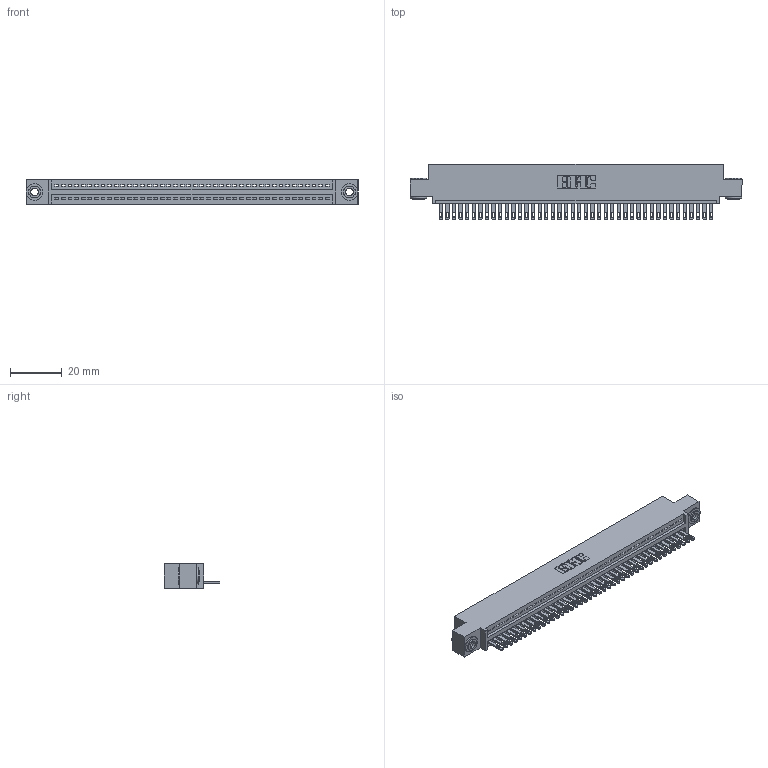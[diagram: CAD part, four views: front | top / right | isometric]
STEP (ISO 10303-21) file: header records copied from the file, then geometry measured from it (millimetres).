
FILE_DESCRIPTION (( 'STEP AP203' ), '1' );
FILE_NAME ('895-042-500-403.STEP', '2020-09-27T01:04:53', ( '' ), ( '' ), 'SwSTEP 2.0', 'SolidWorks 2020', '' );
FILE_SCHEMA (( 'CONFIG_CONTROL_DESIGN' ));
Length unit declared in the file: inch
Products named in the file (4): 845 Part_0.110 Offset - 0.156 Dia-TH; 895-042-500-403; 345-250-002_345-250-002-102; 345-292-001_345-293-100
Assembly tree (45 placements, depth 2):
  895-042-500-403
    845 Part_0.110 Offset - 0.156 Dia-TH
    345-292-001_345-293-100  x42
    345-250-002_345-250-002-102  x2
Bounding box: 127.89 x 21.51 x 9.4 mm (x, y, z)
Volume: 12119.1 mm3; surface area: 16495.8 mm2
Topology: 45 solids, 45 shells, 2436 faces, 7485 edges, 4986 vertices
Faces by surface type: plane 1522, cylinder 906, cone 8
Entity records: 32322 total; most frequent: CARTESIAN_POINT 5577, ORIENTED_EDGE 5546, DIRECTION 4903, EDGE_CURVE 2773, VECTOR 2445, LINE 2445, VERTEX_POINT 1846, AXIS2_PLACEMENT_3D 1229
